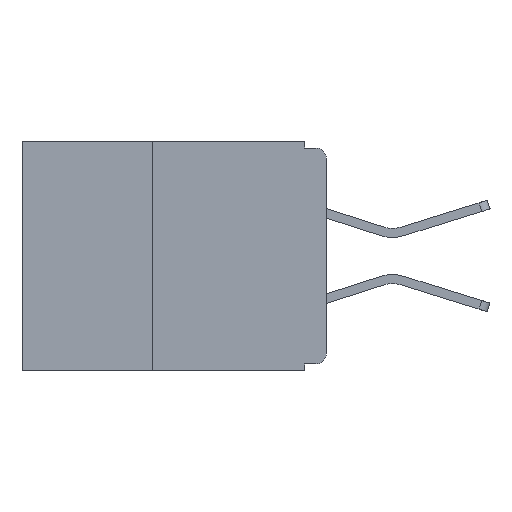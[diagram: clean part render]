
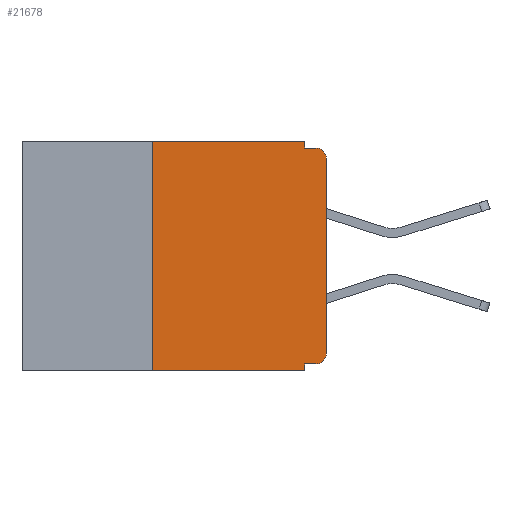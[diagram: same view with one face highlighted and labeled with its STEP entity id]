
A CAD part, left-side view. The second image highlights one B-rep face of the part: STEP entity #21678.
In plain terms, the highlighted planar face has unit normal (-1, 0, 0).
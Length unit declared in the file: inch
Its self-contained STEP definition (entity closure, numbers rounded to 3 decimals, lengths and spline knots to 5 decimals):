
#331 = LINE ( 'NONE', #1685, #14129 ) ;
#541 = ORIENTED_EDGE ( 'NONE', *, *, #33989, .T. ) ;
#587 = VERTEX_POINT ( 'NONE', #7270 ) ;
#679 = CARTESIAN_POINT ( 'NONE',  ( 0., 0.25, -0.33 ) ) ;
#850 = EDGE_LOOP ( 'NONE', ( #28738, #7856, #25847, #20335, #22897, #3542, #33281, #19908, #28773, #541 ) ) ;
#1363 = VECTOR ( 'NONE', #19381, 39.37008 ) ;
#1685 = CARTESIAN_POINT ( 'NONE',  ( 0., 0., -0.32 ) ) ;
#2381 = CARTESIAN_POINT ( 'NONE',  ( 0., 0.25, 0. ) ) ;
#3013 = VERTEX_POINT ( 'NONE', #32319 ) ;
#3091 = LINE ( 'NONE', #16604, #1363 ) ;
#3129 = CARTESIAN_POINT ( 'NONE',  ( 0., 0.015, -0.025 ) ) ;
#3223 = AXIS2_PLACEMENT_3D ( 'NONE', #7137, #23708, #7258 ) ;
#3542 = ORIENTED_EDGE ( 'NONE', *, *, #26673, .F. ) ;
#3937 = LINE ( 'NONE', #33637, #32011 ) ;
#4473 = DIRECTION ( 'NONE',  ( 0., 1., 0. ) ) ;
#4715 = LINE ( 'NONE', #18517, #31906 ) ;
#5523 = CARTESIAN_POINT ( 'NONE',  ( 0., 0.015, -0.305 ) ) ;
#5907 = DIRECTION ( 'NONE',  ( 0., 0., -1. ) ) ;
#6501 = EDGE_CURVE ( 'NONE', #3013, #587, #331, .T. ) ;
#7137 = CARTESIAN_POINT ( 'NONE',  ( 0., 0.437, 0. ) ) ;
#7258 = DIRECTION ( 'NONE',  ( 0., 0., -1. ) ) ;
#7270 = CARTESIAN_POINT ( 'NONE',  ( 0., 0.031, -0.32 ) ) ;
#7856 = ORIENTED_EDGE ( 'NONE', *, *, #27591, .T. ) ;
#7988 = VECTOR ( 'NONE', #11982, 39.37008 ) ;
#8259 = DIRECTION ( 'NONE',  ( 0., 0., -1. ) ) ;
#8617 = VERTEX_POINT ( 'NONE', #679 ) ;
#8862 = LINE ( 'NONE', #9226, #7988 ) ;
#9020 = LINE ( 'NONE', #31744, #22756 ) ;
#9226 = CARTESIAN_POINT ( 'NONE',  ( 0., 0.031, -0.33 ) ) ;
#10319 = VERTEX_POINT ( 'NONE', #29867 ) ;
#10497 = CARTESIAN_POINT ( 'NONE',  ( 0., 0., 0. ) ) ;
#10544 = LINE ( 'NONE', #10497, #24275 ) ;
#10642 = AXIS2_PLACEMENT_3D ( 'NONE', #5523, #24678, #8259 ) ;
#11136 = EDGE_CURVE ( 'NONE', #587, #22116, #8862, .T. ) ;
#11549 = EDGE_CURVE ( 'NONE', #10319, #15640, #10544, .T. ) ;
#11864 = CARTESIAN_POINT ( 'NONE',  ( 0., 0.031, 0. ) ) ;
#11982 = DIRECTION ( 'NONE',  ( 0., 0., -1. ) ) ;
#13255 = DIRECTION ( 'NONE',  ( 0., 0., 1. ) ) ;
#14129 = VECTOR ( 'NONE', #4473, 39.37008 ) ;
#15640 = VERTEX_POINT ( 'NONE', #21123 ) ;
#16604 = CARTESIAN_POINT ( 'NONE',  ( 0., 0.437, -0.33 ) ) ;
#17392 = CIRCLE ( 'NONE', #10642, 0.015 ) ;
#17564 = CARTESIAN_POINT ( 'NONE',  ( 0., 0.031, -0.33 ) ) ;
#18517 = CARTESIAN_POINT ( 'NONE',  ( 0., 0.437, 0. ) ) ;
#19082 = VECTOR ( 'NONE', #26909, 39.37008 ) ;
#19381 = DIRECTION ( 'NONE',  ( 0., -1., 0. ) ) ;
#19908 = ORIENTED_EDGE ( 'NONE', *, *, #11136, .F. ) ;
#19919 = LINE ( 'NONE', #24248, #19082 ) ;
#20068 = VERTEX_POINT ( 'NONE', #27648 ) ;
#20335 = ORIENTED_EDGE ( 'NONE', *, *, #24885, .F. ) ;
#20958 = PLANE ( 'NONE',  #3223 ) ;
#21123 = CARTESIAN_POINT ( 'NONE',  ( 0., 0., -0.025 ) ) ;
#21678 = ADVANCED_FACE ( 'NONE', ( #26491 ), #20958, .F. ) ;
#22095 = VERTEX_POINT ( 'NONE', #33379 ) ;
#22116 = VERTEX_POINT ( 'NONE', #17564 ) ;
#22341 = DIRECTION ( 'NONE',  ( -1., 0., 0. ) ) ;
#22756 = VECTOR ( 'NONE', #34377, 39.37008 ) ;
#22897 = ORIENTED_EDGE ( 'NONE', *, *, #31916, .F. ) ;
#23708 = DIRECTION ( 'NONE',  ( 1., 0., 0. ) ) ;
#24016 = DIRECTION ( 'NONE',  ( 0., -1., 0. ) ) ;
#24248 = CARTESIAN_POINT ( 'NONE',  ( 0., 0., -0.01 ) ) ;
#24275 = VECTOR ( 'NONE', #13255, 39.37008 ) ;
#24678 = DIRECTION ( 'NONE',  ( -1., 0., 0. ) ) ;
#24885 = EDGE_CURVE ( 'NONE', #32266, #20068, #3937, .T. ) ;
#25847 = ORIENTED_EDGE ( 'NONE', *, *, #28853, .F. ) ;
#26491 = FACE_OUTER_BOUND ( 'NONE', #850, .T. ) ;
#26673 = EDGE_CURVE ( 'NONE', #8617, #30814, #9020, .T. ) ;
#26909 = DIRECTION ( 'NONE',  ( 0., -1., 0. ) ) ;
#27308 = CIRCLE ( 'NONE', #32096, 0.015 ) ;
#27591 = EDGE_CURVE ( 'NONE', #15640, #22095, #27308, .T. ) ;
#27648 = CARTESIAN_POINT ( 'NONE',  ( 0., 0.031, -0.01 ) ) ;
#28738 = ORIENTED_EDGE ( 'NONE', *, *, #11549, .T. ) ;
#28773 = ORIENTED_EDGE ( 'NONE', *, *, #6501, .F. ) ;
#28853 = EDGE_CURVE ( 'NONE', #20068, #22095, #19919, .T. ) ;
#29867 = CARTESIAN_POINT ( 'NONE',  ( 0., 0., -0.305 ) ) ;
#30219 = EDGE_CURVE ( 'NONE', #8617, #22116, #3091, .T. ) ;
#30814 = VERTEX_POINT ( 'NONE', #2381 ) ;
#31115 = DIRECTION ( 'NONE',  ( 0., 0., -1. ) ) ;
#31744 = CARTESIAN_POINT ( 'NONE',  ( 0., 0.25, -0.33 ) ) ;
#31906 = VECTOR ( 'NONE', #24016, 39.37008 ) ;
#31916 = EDGE_CURVE ( 'NONE', #30814, #32266, #4715, .T. ) ;
#32011 = VECTOR ( 'NONE', #31115, 39.37008 ) ;
#32096 = AXIS2_PLACEMENT_3D ( 'NONE', #3129, #22341, #5907 ) ;
#32266 = VERTEX_POINT ( 'NONE', #11864 ) ;
#32319 = CARTESIAN_POINT ( 'NONE',  ( 0., 0.015, -0.32 ) ) ;
#33281 = ORIENTED_EDGE ( 'NONE', *, *, #30219, .T. ) ;
#33379 = CARTESIAN_POINT ( 'NONE',  ( 0., 0.015, -0.01 ) ) ;
#33637 = CARTESIAN_POINT ( 'NONE',  ( 0., 0.031, 0. ) ) ;
#33989 = EDGE_CURVE ( 'NONE', #3013, #10319, #17392, .T. ) ;
#34377 = DIRECTION ( 'NONE',  ( 0., 0., 1. ) ) ;
